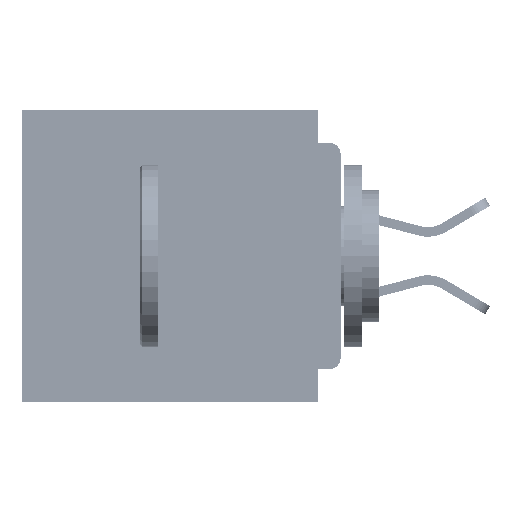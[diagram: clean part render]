
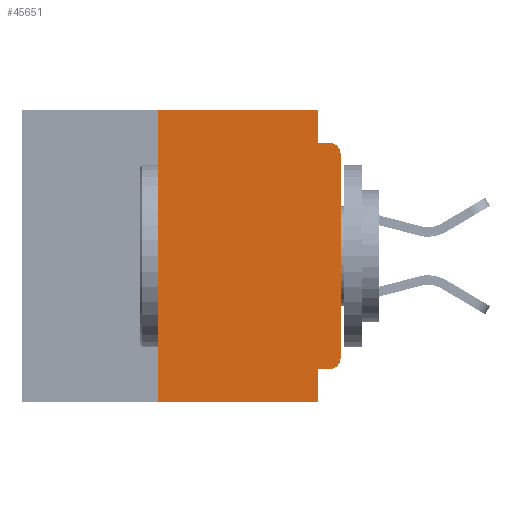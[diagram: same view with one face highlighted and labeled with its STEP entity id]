
A CAD part, left-side view. The second image highlights one B-rep face of the part: STEP entity #45651.
In plain terms, the highlighted planar face has unit normal (-1, 0, 0).
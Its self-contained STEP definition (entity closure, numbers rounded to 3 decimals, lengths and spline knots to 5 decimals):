
#819 = CIRCLE ( 'NONE', #28167, 0.015 ) ;
#1047 = VECTOR ( 'NONE', #17525, 39.37008 ) ;
#1805 = ORIENTED_EDGE ( 'NONE', *, *, #3072, .T. ) ;
#2157 = LINE ( 'NONE', #5961, #27627 ) ;
#2753 = CIRCLE ( 'NONE', #29660, 0.015 ) ;
#2790 = VERTEX_POINT ( 'NONE', #14224 ) ;
#3072 = EDGE_CURVE ( 'NONE', #58331, #56899, #2157, .T. ) ;
#4877 = CARTESIAN_POINT ( 'NONE',  ( 0., 0.015, -0.34 ) ) ;
#5063 = LINE ( 'NONE', #49480, #42312 ) ;
#5431 = EDGE_CURVE ( 'NONE', #44309, #19042, #37575, .T. ) ;
#5961 = CARTESIAN_POINT ( 'NONE',  ( 0., 0.437, -0.4 ) ) ;
#6306 = LINE ( 'NONE', #62315, #34890 ) ;
#7706 = CARTESIAN_POINT ( 'NONE',  ( 0., 0.015, -0.355 ) ) ;
#9679 = CARTESIAN_POINT ( 'NONE',  ( 0., 0., -0.045 ) ) ;
#9742 = ORIENTED_EDGE ( 'NONE', *, *, #42030, .T. ) ;
#9977 = DIRECTION ( 'NONE',  ( 0., 0., -1. ) ) ;
#10482 = EDGE_LOOP ( 'NONE', ( #39582, #9742, #39403, #19809, #13707, #43764, #1805, #48332, #16107, #39729 ) ) ;
#10627 = VECTOR ( 'NONE', #64834, 39.37008 ) ;
#11146 = VERTEX_POINT ( 'NONE', #23710 ) ;
#11221 = CARTESIAN_POINT ( 'NONE',  ( 0., 0.031, -0.4 ) ) ;
#11246 = VERTEX_POINT ( 'NONE', #54263 ) ;
#11994 = LINE ( 'NONE', #49308, #25505 ) ;
#12954 = CARTESIAN_POINT ( 'NONE',  ( 0., 0.031, -0.045 ) ) ;
#13707 = ORIENTED_EDGE ( 'NONE', *, *, #27583, .F. ) ;
#14153 = DIRECTION ( 'NONE',  ( 0., 0., 1. ) ) ;
#14224 = CARTESIAN_POINT ( 'NONE',  ( 0., 0., -0.06 ) ) ;
#14572 = VECTOR ( 'NONE', #46629, 39.37008 ) ;
#14630 = LINE ( 'NONE', #22394, #1047 ) ;
#16107 = ORIENTED_EDGE ( 'NONE', *, *, #62079, .F. ) ;
#16642 = VERTEX_POINT ( 'NONE', #18403 ) ;
#17227 = EDGE_CURVE ( 'NONE', #11246, #44309, #14630, .T. ) ;
#17444 = EDGE_CURVE ( 'NONE', #58331, #16642, #5063, .T. ) ;
#17525 = DIRECTION ( 'NONE',  ( 0., 0., -1. ) ) ;
#17705 = EDGE_CURVE ( 'NONE', #11146, #56899, #41493, .T. ) ;
#18403 = CARTESIAN_POINT ( 'NONE',  ( 0., 0.25, 0. ) ) ;
#19008 = VERTEX_POINT ( 'NONE', #26379 ) ;
#19042 = VERTEX_POINT ( 'NONE', #51675 ) ;
#19084 = DIRECTION ( 'NONE',  ( 0., 1., 0. ) ) ;
#19809 = ORIENTED_EDGE ( 'NONE', *, *, #17227, .F. ) ;
#21308 = AXIS2_PLACEMENT_3D ( 'NONE', #55118, #25014, #60102 ) ;
#22304 = VECTOR ( 'NONE', #26688, 39.37008 ) ;
#22394 = CARTESIAN_POINT ( 'NONE',  ( 0., 0.031, 0. ) ) ;
#23710 = CARTESIAN_POINT ( 'NONE',  ( 0., 0.031, -0.355 ) ) ;
#25014 = DIRECTION ( 'NONE',  ( 1., 0., 0. ) ) ;
#25505 = VECTOR ( 'NONE', #19084, 39.37008 ) ;
#26379 = CARTESIAN_POINT ( 'NONE',  ( 0., 0., -0.34 ) ) ;
#26688 = DIRECTION ( 'NONE',  ( 0., 0., 1. ) ) ;
#26730 = DIRECTION ( 'NONE',  ( -1., 0., 0. ) ) ;
#26865 = EDGE_CURVE ( 'NONE', #19008, #2790, #49138, .T. ) ;
#27583 = EDGE_CURVE ( 'NONE', #16642, #11246, #6306, .T. ) ;
#27627 = VECTOR ( 'NONE', #41201, 39.37008 ) ;
#28167 = AXIS2_PLACEMENT_3D ( 'NONE', #4877, #40342, #9977 ) ;
#29327 = CARTESIAN_POINT ( 'NONE',  ( 0., 0.031, -0.4 ) ) ;
#29660 = AXIS2_PLACEMENT_3D ( 'NONE', #56801, #26730, #61765 ) ;
#34890 = VECTOR ( 'NONE', #37427, 39.37008 ) ;
#36048 = EDGE_CURVE ( 'NONE', #49353, #19008, #819, .T. ) ;
#37427 = DIRECTION ( 'NONE',  ( 0., -1., 0. ) ) ;
#37575 = LINE ( 'NONE', #9679, #10627 ) ;
#39403 = ORIENTED_EDGE ( 'NONE', *, *, #5431, .F. ) ;
#39582 = ORIENTED_EDGE ( 'NONE', *, *, #26865, .T. ) ;
#39729 = ORIENTED_EDGE ( 'NONE', *, *, #36048, .T. ) ;
#40342 = DIRECTION ( 'NONE',  ( -1., 0., 0. ) ) ;
#41201 = DIRECTION ( 'NONE',  ( 0., -1., 0. ) ) ;
#41493 = LINE ( 'NONE', #11221, #14572 ) ;
#42030 = EDGE_CURVE ( 'NONE', #2790, #19042, #2753, .T. ) ;
#42312 = VECTOR ( 'NONE', #14153, 39.37008 ) ;
#43764 = ORIENTED_EDGE ( 'NONE', *, *, #17444, .F. ) ;
#44309 = VERTEX_POINT ( 'NONE', #12954 ) ;
#45651 = ADVANCED_FACE ( 'NONE', ( #63393 ), #50130, .F. ) ;
#46629 = DIRECTION ( 'NONE',  ( 0., 0., -1. ) ) ;
#48332 = ORIENTED_EDGE ( 'NONE', *, *, #17705, .F. ) ;
#49138 = LINE ( 'NONE', #51994, #22304 ) ;
#49308 = CARTESIAN_POINT ( 'NONE',  ( 0., 0., -0.355 ) ) ;
#49353 = VERTEX_POINT ( 'NONE', #7706 ) ;
#49480 = CARTESIAN_POINT ( 'NONE',  ( 0., 0.25, -0.4 ) ) ;
#50130 = PLANE ( 'NONE',  #21308 ) ;
#51675 = CARTESIAN_POINT ( 'NONE',  ( 0., 0.015, -0.045 ) ) ;
#51994 = CARTESIAN_POINT ( 'NONE',  ( 0., 0., 0. ) ) ;
#53156 = CARTESIAN_POINT ( 'NONE',  ( 0., 0.25, -0.4 ) ) ;
#54263 = CARTESIAN_POINT ( 'NONE',  ( 0., 0.031, 0. ) ) ;
#55118 = CARTESIAN_POINT ( 'NONE',  ( 0., 0.437, 0. ) ) ;
#56801 = CARTESIAN_POINT ( 'NONE',  ( 0., 0.015, -0.06 ) ) ;
#56899 = VERTEX_POINT ( 'NONE', #29327 ) ;
#58331 = VERTEX_POINT ( 'NONE', #53156 ) ;
#60102 = DIRECTION ( 'NONE',  ( 0., 0., -1. ) ) ;
#61765 = DIRECTION ( 'NONE',  ( 0., 0., -1. ) ) ;
#62079 = EDGE_CURVE ( 'NONE', #49353, #11146, #11994, .T. ) ;
#62315 = CARTESIAN_POINT ( 'NONE',  ( 0., 0.437, 0. ) ) ;
#63393 = FACE_OUTER_BOUND ( 'NONE', #10482, .T. ) ;
#64834 = DIRECTION ( 'NONE',  ( 0., -1., 0. ) ) ;
